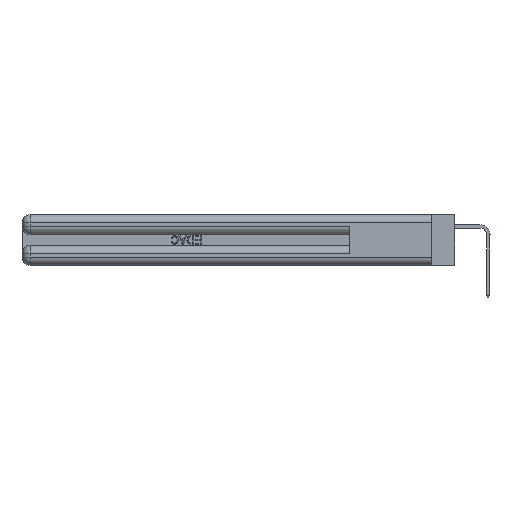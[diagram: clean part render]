
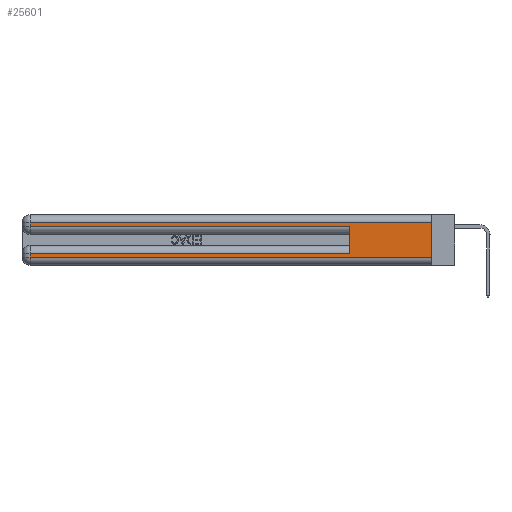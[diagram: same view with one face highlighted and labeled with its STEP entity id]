
A CAD part, left-side view. The second image highlights one B-rep face of the part: STEP entity #25601.
In plain terms, the highlighted planar face has unit normal (-1, 0, 0).
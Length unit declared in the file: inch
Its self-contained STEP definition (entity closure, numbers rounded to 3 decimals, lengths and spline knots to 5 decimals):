
#223 = DIRECTION ( 'NONE',  ( 0., 0., 1. ) ) ;
#1007 = LINE ( 'NONE', #4143, #17990 ) ;
#3792 = LINE ( 'NONE', #5935, #38724 ) ;
#4143 = CARTESIAN_POINT ( 'NONE',  ( 0., 0., 0.37 ) ) ;
#4936 = LINE ( 'NONE', #34801, #39865 ) ;
#4996 = VERTEX_POINT ( 'NONE', #8801 ) ;
#5272 = CARTESIAN_POINT ( 'NONE',  ( 0., 2.94, 0.31 ) ) ;
#5469 = EDGE_CURVE ( 'NONE', #4996, #15440, #4936, .T. ) ;
#5935 = CARTESIAN_POINT ( 'NONE',  ( 0., 0., 0.285 ) ) ;
#6276 = EDGE_CURVE ( 'NONE', #10413, #21103, #3792, .T. ) ;
#7524 = CARTESIAN_POINT ( 'NONE',  ( 0., 0.6, 0.285 ) ) ;
#7819 = LINE ( 'NONE', #34288, #25866 ) ;
#8801 = CARTESIAN_POINT ( 'NONE',  ( 0., 2.94, 0.085 ) ) ;
#9454 = CARTESIAN_POINT ( 'NONE',  ( 0., 0., 0.06 ) ) ;
#10159 = CARTESIAN_POINT ( 'NONE',  ( 0., 2.94, 0.37 ) ) ;
#10413 = VERTEX_POINT ( 'NONE', #34245 ) ;
#10443 = LINE ( 'NONE', #13714, #37423 ) ;
#10536 = ORIENTED_EDGE ( 'NONE', *, *, #6276, .T. ) ;
#10573 = ORIENTED_EDGE ( 'NONE', *, *, #5469, .T. ) ;
#10682 = EDGE_LOOP ( 'NONE', ( #36898, #32720, #38701, #10536, #21595, #34867, #10573, #20351 ) ) ;
#11630 = LINE ( 'NONE', #10159, #19617 ) ;
#12610 = VERTEX_POINT ( 'NONE', #5272 ) ;
#12633 = CARTESIAN_POINT ( 'NONE',  ( 0., 0., 0.06 ) ) ;
#13594 = DIRECTION ( 'NONE',  ( 0., 0., -1. ) ) ;
#13714 = CARTESIAN_POINT ( 'NONE',  ( 0., 0.6, 0.145 ) ) ;
#14080 = DIRECTION ( 'NONE',  ( 0., 1., 0. ) ) ;
#14393 = DIRECTION ( 'NONE',  ( 0., 0., -1. ) ) ;
#14534 = FACE_OUTER_BOUND ( 'NONE', #10682, .T. ) ;
#15440 = VERTEX_POINT ( 'NONE', #24414 ) ;
#15607 = EDGE_CURVE ( 'NONE', #15815, #4996, #25437, .T. ) ;
#15815 = VERTEX_POINT ( 'NONE', #32918 ) ;
#17769 = LINE ( 'NONE', #12633, #34644 ) ;
#17990 = VECTOR ( 'NONE', #14393, 39.37008 ) ;
#18547 = CARTESIAN_POINT ( 'NONE',  ( 0., 0., 0.37 ) ) ;
#18695 = DIRECTION ( 'NONE',  ( 0., 0., -1. ) ) ;
#19473 = DIRECTION ( 'NONE',  ( 0., -1., 0. ) ) ;
#19617 = VECTOR ( 'NONE', #13594, 39.37008 ) ;
#20351 = ORIENTED_EDGE ( 'NONE', *, *, #25130, .T. ) ;
#21103 = VERTEX_POINT ( 'NONE', #7524 ) ;
#21104 = EDGE_CURVE ( 'NONE', #28654, #28927, #1007, .T. ) ;
#21562 = EDGE_CURVE ( 'NONE', #12610, #10413, #11630, .T. ) ;
#21595 = ORIENTED_EDGE ( 'NONE', *, *, #33050, .F. ) ;
#24414 = CARTESIAN_POINT ( 'NONE',  ( 0., 2.94, 0.06 ) ) ;
#24779 = DIRECTION ( 'NONE',  ( 0., 0., -1. ) ) ;
#25130 = EDGE_CURVE ( 'NONE', #15440, #28927, #17769, .T. ) ;
#25437 = LINE ( 'NONE', #28701, #34410 ) ;
#25601 = ADVANCED_FACE ( 'NONE', ( #14534 ), #35484, .F. ) ;
#25866 = VECTOR ( 'NONE', #14080, 39.37008 ) ;
#28654 = VERTEX_POINT ( 'NONE', #38489 ) ;
#28701 = CARTESIAN_POINT ( 'NONE',  ( 0., 0., 0.085 ) ) ;
#28927 = VERTEX_POINT ( 'NONE', #9454 ) ;
#32051 = DIRECTION ( 'NONE',  ( 0., 1., 0. ) ) ;
#32720 = ORIENTED_EDGE ( 'NONE', *, *, #39025, .T. ) ;
#32918 = CARTESIAN_POINT ( 'NONE',  ( 0., 0.6, 0.085 ) ) ;
#33050 = EDGE_CURVE ( 'NONE', #15815, #21103, #10443, .T. ) ;
#34245 = CARTESIAN_POINT ( 'NONE',  ( 0., 2.94, 0.285 ) ) ;
#34288 = CARTESIAN_POINT ( 'NONE',  ( 0., 0., 0.31 ) ) ;
#34410 = VECTOR ( 'NONE', #32051, 39.37008 ) ;
#34644 = VECTOR ( 'NONE', #19473, 39.37008 ) ;
#34801 = CARTESIAN_POINT ( 'NONE',  ( 0., 2.94, 0.37 ) ) ;
#34867 = ORIENTED_EDGE ( 'NONE', *, *, #15607, .T. ) ;
#35484 = PLANE ( 'NONE',  #37969 ) ;
#36898 = ORIENTED_EDGE ( 'NONE', *, *, #21104, .F. ) ;
#37423 = VECTOR ( 'NONE', #223, 39.37008 ) ;
#37969 = AXIS2_PLACEMENT_3D ( 'NONE', #18547, #38913, #18695 ) ;
#38489 = CARTESIAN_POINT ( 'NONE',  ( 0., 0., 0.31 ) ) ;
#38701 = ORIENTED_EDGE ( 'NONE', *, *, #21562, .T. ) ;
#38724 = VECTOR ( 'NONE', #39806, 39.37008 ) ;
#38913 = DIRECTION ( 'NONE',  ( 1., 0., 0. ) ) ;
#39025 = EDGE_CURVE ( 'NONE', #28654, #12610, #7819, .T. ) ;
#39806 = DIRECTION ( 'NONE',  ( 0., -1., 0. ) ) ;
#39865 = VECTOR ( 'NONE', #24779, 39.37008 ) ;
